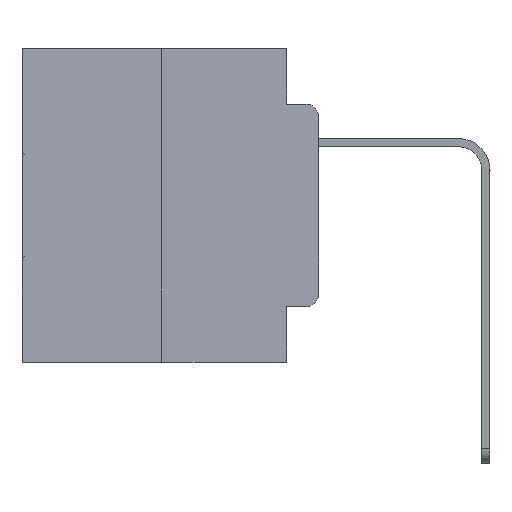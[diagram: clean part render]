
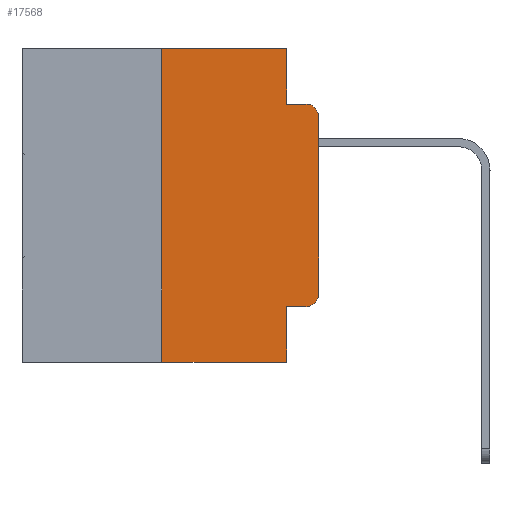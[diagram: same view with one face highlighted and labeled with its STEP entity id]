
A CAD part, left-side view. The second image highlights one B-rep face of the part: STEP entity #17568.
In plain terms, the highlighted planar face has unit normal (-1, 0, 0).
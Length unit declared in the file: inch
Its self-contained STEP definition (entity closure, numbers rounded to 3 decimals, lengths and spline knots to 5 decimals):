
#118 = CARTESIAN_POINT ( 'NONE',  ( 0., 0.051, 0. ) ) ;
#196 = PLANE ( 'NONE',  #22144 ) ;
#387 = CARTESIAN_POINT ( 'NONE',  ( 0., 0.051, -0.0885 ) ) ;
#1529 = VECTOR ( 'NONE', #23067, 39.37008 ) ;
#1671 = EDGE_CURVE ( 'NONE', #23085, #24851, #8365, .T. ) ;
#2188 = ORIENTED_EDGE ( 'NONE', *, *, #20930, .F. ) ;
#3191 = VERTEX_POINT ( 'NONE', #3396 ) ;
#3349 = CARTESIAN_POINT ( 'NONE',  ( 0., 0.25, 0. ) ) ;
#3396 = CARTESIAN_POINT ( 'NONE',  ( 0., 0.02, -0.0885 ) ) ;
#4329 = EDGE_CURVE ( 'NONE', #28466, #7711, #11419, .T. ) ;
#4401 = ORIENTED_EDGE ( 'NONE', *, *, #12902, .T. ) ;
#4735 = DIRECTION ( 'NONE',  ( 1., 0., 0. ) ) ;
#5300 = LINE ( 'NONE', #6444, #6012 ) ;
#5541 = CARTESIAN_POINT ( 'NONE',  ( 0., 0.051, 0. ) ) ;
#5775 = CARTESIAN_POINT ( 'NONE',  ( 0., 0., -0.1085 ) ) ;
#5970 = DIRECTION ( 'NONE',  ( 0., -1., 0. ) ) ;
#6012 = VECTOR ( 'NONE', #12720, 39.37008 ) ;
#6444 = CARTESIAN_POINT ( 'NONE',  ( 0., 0.25, 0. ) ) ;
#6617 = ORIENTED_EDGE ( 'NONE', *, *, #18189, .F. ) ;
#6835 = EDGE_LOOP ( 'NONE', ( #28791, #17755, #9185, #21895, #6617, #21271, #28252, #2188, #4401, #27629 ) ) ;
#7082 = VECTOR ( 'NONE', #27303, 39.37008 ) ;
#7149 = CARTESIAN_POINT ( 'NONE',  ( 0., 0.02, -0.1085 ) ) ;
#7711 = VERTEX_POINT ( 'NONE', #5775 ) ;
#8365 = LINE ( 'NONE', #10774, #12932 ) ;
#8415 = VECTOR ( 'NONE', #5970, 39.37008 ) ;
#9185 = ORIENTED_EDGE ( 'NONE', *, *, #23594, .F. ) ;
#9249 = CARTESIAN_POINT ( 'NONE',  ( 0., 0.051, -0.5 ) ) ;
#9402 = CARTESIAN_POINT ( 'NONE',  ( 0., 0., 0. ) ) ;
#10308 = CARTESIAN_POINT ( 'NONE',  ( 0., 0.051, -0.4115 ) ) ;
#10375 = CARTESIAN_POINT ( 'NONE',  ( 0., 0., -0.3915 ) ) ;
#10774 = CARTESIAN_POINT ( 'NONE',  ( 0., 0.051, 0. ) ) ;
#10907 = VECTOR ( 'NONE', #18083, 39.37008 ) ;
#11277 = CIRCLE ( 'NONE', #23806, 0.02 ) ;
#11419 = LINE ( 'NONE', #9402, #1529 ) ;
#11479 = CARTESIAN_POINT ( 'NONE',  ( 0., 0.473, 0. ) ) ;
#11561 = CARTESIAN_POINT ( 'NONE',  ( 0., 0.051, -0.0885 ) ) ;
#12472 = CARTESIAN_POINT ( 'NONE',  ( 0., 0.02, -0.3915 ) ) ;
#12720 = DIRECTION ( 'NONE',  ( 0., 0., 1. ) ) ;
#12902 = EDGE_CURVE ( 'NONE', #13730, #18504, #22837, .T. ) ;
#12932 = VECTOR ( 'NONE', #15491, 39.37008 ) ;
#13614 = DIRECTION ( 'NONE',  ( 0., 0., -1. ) ) ;
#13730 = VERTEX_POINT ( 'NONE', #22170 ) ;
#14054 = VERTEX_POINT ( 'NONE', #3349 ) ;
#14840 = DIRECTION ( 'NONE',  ( 0., 0., -1. ) ) ;
#15491 = DIRECTION ( 'NONE',  ( 0., 0., -1. ) ) ;
#15555 = AXIS2_PLACEMENT_3D ( 'NONE', #12472, #17028, #14840 ) ;
#15807 = DIRECTION ( 'NONE',  ( -1., 0., 0. ) ) ;
#15953 = CARTESIAN_POINT ( 'NONE',  ( 0., 0.473, 0. ) ) ;
#17028 = DIRECTION ( 'NONE',  ( -1., 0., 0. ) ) ;
#17264 = LINE ( 'NONE', #27031, #10907 ) ;
#17568 = ADVANCED_FACE ( 'NONE', ( #24410 ), #196, .F. ) ;
#17755 = ORIENTED_EDGE ( 'NONE', *, *, #19551, .T. ) ;
#17969 = EDGE_CURVE ( 'NONE', #18504, #28466, #25454, .T. ) ;
#18044 = LINE ( 'NONE', #11479, #26461 ) ;
#18083 = DIRECTION ( 'NONE',  ( 0., -1., 0. ) ) ;
#18189 = EDGE_CURVE ( 'NONE', #14054, #23085, #18044, .T. ) ;
#18504 = VERTEX_POINT ( 'NONE', #25935 ) ;
#19551 = EDGE_CURVE ( 'NONE', #7711, #3191, #11277, .T. ) ;
#19584 = EDGE_CURVE ( 'NONE', #25835, #24846, #17264, .T. ) ;
#20493 = DIRECTION ( 'NONE',  ( 0., 0., -1. ) ) ;
#20533 = DIRECTION ( 'NONE',  ( 0., 0., -1. ) ) ;
#20930 = EDGE_CURVE ( 'NONE', #13730, #24846, #28784, .T. ) ;
#21271 = ORIENTED_EDGE ( 'NONE', *, *, #23807, .F. ) ;
#21895 = ORIENTED_EDGE ( 'NONE', *, *, #1671, .F. ) ;
#22144 = AXIS2_PLACEMENT_3D ( 'NONE', #15953, #4735, #20493 ) ;
#22170 = CARTESIAN_POINT ( 'NONE',  ( 0., 0.051, -0.4115 ) ) ;
#22789 = DIRECTION ( 'NONE',  ( 0., -1., 0. ) ) ;
#22837 = LINE ( 'NONE', #10308, #8415 ) ;
#23067 = DIRECTION ( 'NONE',  ( 0., 0., 1. ) ) ;
#23085 = VERTEX_POINT ( 'NONE', #5541 ) ;
#23267 = LINE ( 'NONE', #11561, #7082 ) ;
#23594 = EDGE_CURVE ( 'NONE', #24851, #3191, #23267, .T. ) ;
#23806 = AXIS2_PLACEMENT_3D ( 'NONE', #7149, #15807, #20533 ) ;
#23807 = EDGE_CURVE ( 'NONE', #25835, #14054, #5300, .T. ) ;
#24410 = FACE_OUTER_BOUND ( 'NONE', #6835, .T. ) ;
#24846 = VERTEX_POINT ( 'NONE', #9249 ) ;
#24851 = VERTEX_POINT ( 'NONE', #387 ) ;
#25454 = CIRCLE ( 'NONE', #15555, 0.02 ) ;
#25835 = VERTEX_POINT ( 'NONE', #26728 ) ;
#25935 = CARTESIAN_POINT ( 'NONE',  ( 0., 0.02, -0.4115 ) ) ;
#26355 = VECTOR ( 'NONE', #13614, 39.37008 ) ;
#26461 = VECTOR ( 'NONE', #22789, 39.37008 ) ;
#26728 = CARTESIAN_POINT ( 'NONE',  ( 0., 0.25, -0.5 ) ) ;
#27031 = CARTESIAN_POINT ( 'NONE',  ( 0., 0.473, -0.5 ) ) ;
#27303 = DIRECTION ( 'NONE',  ( 0., -1., 0. ) ) ;
#27629 = ORIENTED_EDGE ( 'NONE', *, *, #17969, .T. ) ;
#28252 = ORIENTED_EDGE ( 'NONE', *, *, #19584, .T. ) ;
#28466 = VERTEX_POINT ( 'NONE', #10375 ) ;
#28784 = LINE ( 'NONE', #118, #26355 ) ;
#28791 = ORIENTED_EDGE ( 'NONE', *, *, #4329, .T. ) ;
